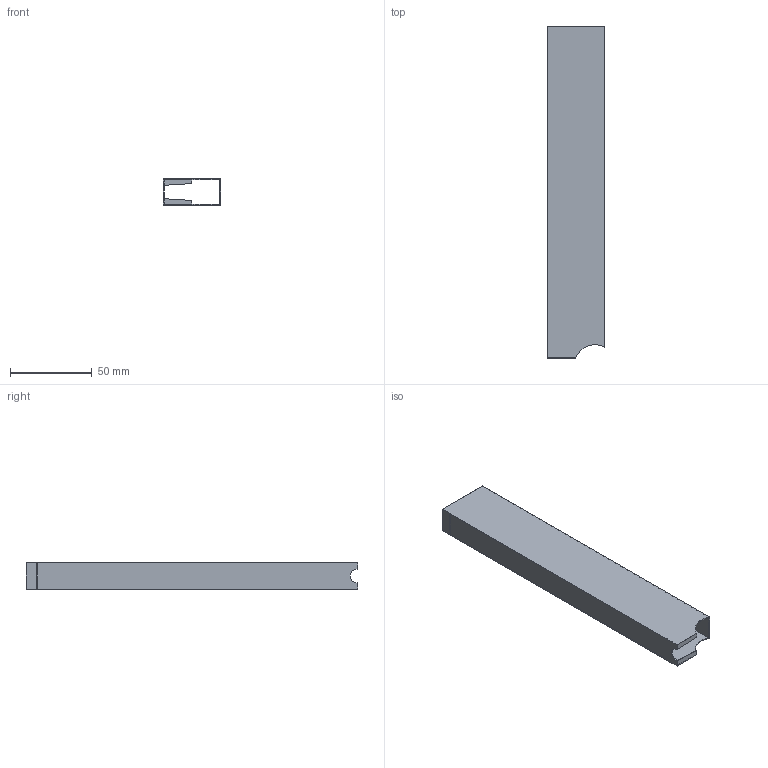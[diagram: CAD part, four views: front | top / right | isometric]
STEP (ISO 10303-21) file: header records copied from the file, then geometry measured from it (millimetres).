
FILE_DESCRIPTION (( 'STEP AP214' ), '1' );
FILE_NAME ('SHUTY_MAG.STEP', '2013-05-15T15:00:57', ( 'Asher' ), ( '' ), 'SwSTEP 2.0', 'SolidWorks 2013', '' );
FILE_SCHEMA (( 'AUTOMOTIVE_DESIGN' ));
Length unit declared in the file: inch
Products named in the file (1): SHUTY_MAG
Bounding box: 35 x 203.2 x 16 mm (x, y, z)
Volume: 10178.6 mm3; surface area: 40202.9 mm2
Topology: 1 solids, 1 shells, 28 faces, 78 edges, 50 vertices
Faces by surface type: plane 26, cylinder 2
Entity records: 932 total; most frequent: CARTESIAN_POINT 157, ORIENTED_EDGE 156, DIRECTION 142, EDGE_CURVE 78, LINE 72, VECTOR 72, VERTEX_POINT 50, AXIS2_PLACEMENT_3D 35
